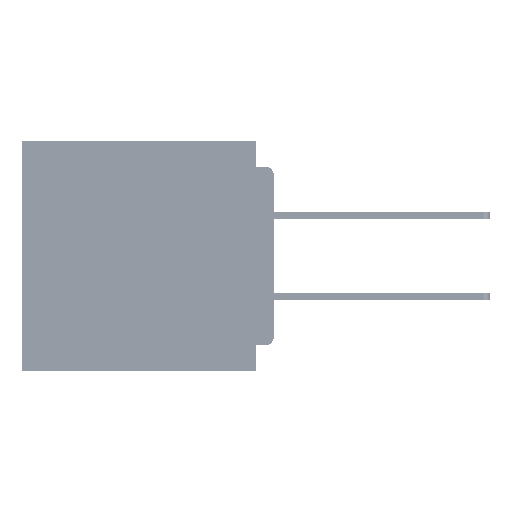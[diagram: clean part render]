
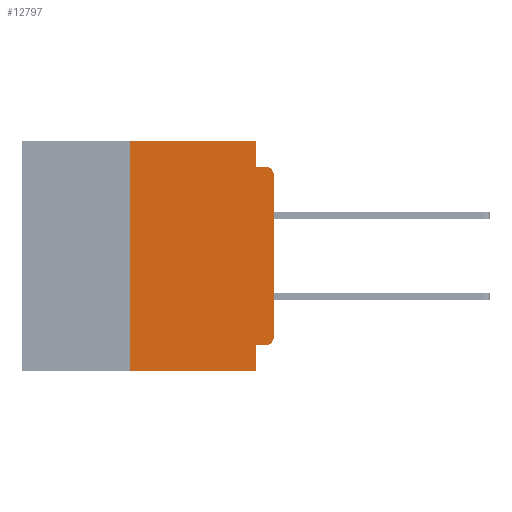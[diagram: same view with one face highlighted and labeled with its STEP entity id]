
A CAD part, left-side view. The second image highlights one B-rep face of the part: STEP entity #12797.
In plain terms, the highlighted planar face has unit normal (-1, 0, 0).
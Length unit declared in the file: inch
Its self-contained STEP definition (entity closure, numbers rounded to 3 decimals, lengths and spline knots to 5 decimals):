
#706 = CARTESIAN_POINT ( 'NONE',  ( 0., 0.25, 0. ) ) ;
#2493 = CARTESIAN_POINT ( 'NONE',  ( 0., 0.031, -0.4 ) ) ;
#3553 = VERTEX_POINT ( 'NONE', #52940 ) ;
#4804 = DIRECTION ( 'NONE',  ( 0., 0., 1. ) ) ;
#6430 = PLANE ( 'NONE',  #67589 ) ;
#8992 = CARTESIAN_POINT ( 'NONE',  ( 0., 0., -0.355 ) ) ;
#10153 = CARTESIAN_POINT ( 'NONE',  ( 0., 0.25, -0.4 ) ) ;
#10250 = ORIENTED_EDGE ( 'NONE', *, *, #67132, .T. ) ;
#11442 = ORIENTED_EDGE ( 'NONE', *, *, #51162, .T. ) ;
#11752 = CARTESIAN_POINT ( 'NONE',  ( 0., 0.437, 0. ) ) ;
#11986 = DIRECTION ( 'NONE',  ( 0., 0., -1. ) ) ;
#12796 = LINE ( 'NONE', #26063, #66978 ) ;
#12797 = ADVANCED_FACE ( 'NONE', ( #67858 ), #6430, .F. ) ;
#14764 = CIRCLE ( 'NONE', #17972, 0.015 ) ;
#15019 = VECTOR ( 'NONE', #36829, 39.37008 ) ;
#15590 = VERTEX_POINT ( 'NONE', #706 ) ;
#16935 = DIRECTION ( 'NONE',  ( 0., 0., -1. ) ) ;
#17002 = CARTESIAN_POINT ( 'NONE',  ( 0., 0.031, -0.355 ) ) ;
#17016 = DIRECTION ( 'NONE',  ( 1., 0., 0. ) ) ;
#17292 = DIRECTION ( 'NONE',  ( -1., 0., 0. ) ) ;
#17972 = AXIS2_PLACEMENT_3D ( 'NONE', #30801, #67509, #36104 ) ;
#19179 = LINE ( 'NONE', #10153, #59480 ) ;
#21571 = EDGE_CURVE ( 'NONE', #66496, #64554, #12796, .T. ) ;
#23783 = LINE ( 'NONE', #53694, #64035 ) ;
#24564 = DIRECTION ( 'NONE',  ( 0., 1., 0. ) ) ;
#26063 = CARTESIAN_POINT ( 'NONE',  ( 0., 0., -0.045 ) ) ;
#27109 = VERTEX_POINT ( 'NONE', #60844 ) ;
#28311 = CARTESIAN_POINT ( 'NONE',  ( 0., 0., -0.34 ) ) ;
#29378 = CARTESIAN_POINT ( 'NONE',  ( 0., 0., -0.06 ) ) ;
#29957 = VERTEX_POINT ( 'NONE', #29378 ) ;
#30394 = ORIENTED_EDGE ( 'NONE', *, *, #57070, .F. ) ;
#30664 = LINE ( 'NONE', #62932, #15019 ) ;
#30801 = CARTESIAN_POINT ( 'NONE',  ( 0., 0.015, -0.34 ) ) ;
#32582 = VERTEX_POINT ( 'NONE', #65581 ) ;
#33529 = LINE ( 'NONE', #64519, #59820 ) ;
#35583 = ORIENTED_EDGE ( 'NONE', *, *, #54804, .T. ) ;
#36104 = DIRECTION ( 'NONE',  ( 0., 0., -1. ) ) ;
#36257 = EDGE_CURVE ( 'NONE', #32582, #44523, #60984, .T. ) ;
#36829 = DIRECTION ( 'NONE',  ( 0., -1., 0. ) ) ;
#37267 = VERTEX_POINT ( 'NONE', #28311 ) ;
#37382 = EDGE_CURVE ( 'NONE', #15590, #3553, #49033, .T. ) ;
#37567 = LINE ( 'NONE', #45547, #63774 ) ;
#42472 = ORIENTED_EDGE ( 'NONE', *, *, #66754, .T. ) ;
#42895 = ORIENTED_EDGE ( 'NONE', *, *, #58250, .F. ) ;
#44352 = EDGE_CURVE ( 'NONE', #27109, #15590, #19179, .T. ) ;
#44523 = VERTEX_POINT ( 'NONE', #17002 ) ;
#45547 = CARTESIAN_POINT ( 'NONE',  ( 0., 0., 0. ) ) ;
#46004 = AXIS2_PLACEMENT_3D ( 'NONE', #48746, #17292, #54058 ) ;
#46140 = ORIENTED_EDGE ( 'NONE', *, *, #36257, .F. ) ;
#46732 = CARTESIAN_POINT ( 'NONE',  ( 0., 0.031, -0.045 ) ) ;
#47215 = DIRECTION ( 'NONE',  ( 0., -1., 0. ) ) ;
#47376 = VECTOR ( 'NONE', #65958, 39.37008 ) ;
#48746 = CARTESIAN_POINT ( 'NONE',  ( 0., 0.015, -0.06 ) ) ;
#49033 = LINE ( 'NONE', #60701, #47376 ) ;
#50356 = VECTOR ( 'NONE', #24564, 39.37008 ) ;
#51162 = EDGE_CURVE ( 'NONE', #27109, #51438, #30664, .T. ) ;
#51438 = VERTEX_POINT ( 'NONE', #2493 ) ;
#52940 = CARTESIAN_POINT ( 'NONE',  ( 0., 0.031, 0. ) ) ;
#53532 = ORIENTED_EDGE ( 'NONE', *, *, #37382, .F. ) ;
#53694 = CARTESIAN_POINT ( 'NONE',  ( 0., 0.031, -0.4 ) ) ;
#53777 = DIRECTION ( 'NONE',  ( 0., 0., -1. ) ) ;
#54058 = DIRECTION ( 'NONE',  ( 0., 0., -1. ) ) ;
#54804 = EDGE_CURVE ( 'NONE', #37267, #29957, #37567, .T. ) ;
#55158 = ORIENTED_EDGE ( 'NONE', *, *, #44352, .F. ) ;
#56150 = DIRECTION ( 'NONE',  ( 0., 0., 1. ) ) ;
#57070 = EDGE_CURVE ( 'NONE', #44523, #51438, #23783, .T. ) ;
#58250 = EDGE_CURVE ( 'NONE', #3553, #66496, #33529, .T. ) ;
#59480 = VECTOR ( 'NONE', #4804, 39.37008 ) ;
#59820 = VECTOR ( 'NONE', #11986, 39.37008 ) ;
#60701 = CARTESIAN_POINT ( 'NONE',  ( 0., 0.437, 0. ) ) ;
#60844 = CARTESIAN_POINT ( 'NONE',  ( 0., 0.25, -0.4 ) ) ;
#60984 = LINE ( 'NONE', #8992, #50356 ) ;
#61163 = CARTESIAN_POINT ( 'NONE',  ( 0., 0.015, -0.045 ) ) ;
#62932 = CARTESIAN_POINT ( 'NONE',  ( 0., 0.437, -0.4 ) ) ;
#63774 = VECTOR ( 'NONE', #56150, 39.37008 ) ;
#64035 = VECTOR ( 'NONE', #16935, 39.37008 ) ;
#64519 = CARTESIAN_POINT ( 'NONE',  ( 0., 0.031, 0. ) ) ;
#64554 = VERTEX_POINT ( 'NONE', #61163 ) ;
#65581 = CARTESIAN_POINT ( 'NONE',  ( 0., 0.015, -0.355 ) ) ;
#65748 = CIRCLE ( 'NONE', #46004, 0.015 ) ;
#65958 = DIRECTION ( 'NONE',  ( 0., -1., 0. ) ) ;
#66496 = VERTEX_POINT ( 'NONE', #46732 ) ;
#66754 = EDGE_CURVE ( 'NONE', #29957, #64554, #65748, .T. ) ;
#66978 = VECTOR ( 'NONE', #47215, 39.37008 ) ;
#67121 = EDGE_LOOP ( 'NONE', ( #35583, #42472, #67249, #42895, #53532, #55158, #11442, #30394, #46140, #10250 ) ) ;
#67132 = EDGE_CURVE ( 'NONE', #32582, #37267, #14764, .T. ) ;
#67249 = ORIENTED_EDGE ( 'NONE', *, *, #21571, .F. ) ;
#67509 = DIRECTION ( 'NONE',  ( -1., 0., 0. ) ) ;
#67589 = AXIS2_PLACEMENT_3D ( 'NONE', #11752, #17016, #53777 ) ;
#67858 = FACE_OUTER_BOUND ( 'NONE', #67121, .T. ) ;
